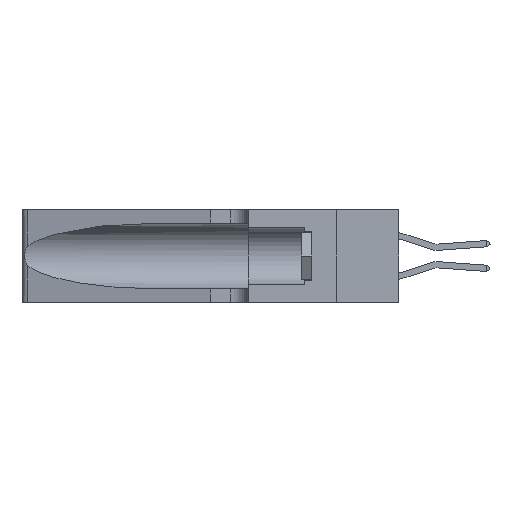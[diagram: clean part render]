
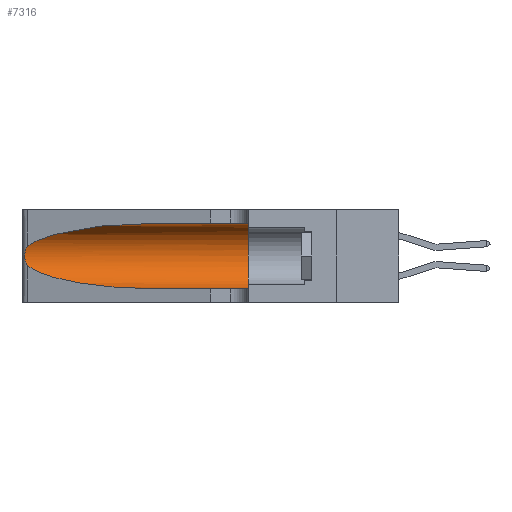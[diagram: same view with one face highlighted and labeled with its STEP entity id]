
A CAD part, left-side view. The second image highlights one B-rep face of the part: STEP entity #7316.
In plain terms, the highlighted cylindrical face has radius 3.308 mm (diameter 6.617 mm), a partial arc.
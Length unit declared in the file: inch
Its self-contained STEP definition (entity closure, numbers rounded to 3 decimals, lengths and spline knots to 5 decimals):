
#1073 = ORIENTED_EDGE ( 'NONE', *, *, #15432, .T. ) ;
#1999 = CARTESIAN_POINT ( 'NONE',  ( 0.25639, 1.23184, 0.21858 ) ) ;
#2359 = VERTEX_POINT ( 'NONE', #31182 ) ;
#3032 = EDGE_CURVE ( 'NONE', #23920, #23145, #36946, .T. ) ;
#3765 = EDGE_LOOP ( 'NONE', ( #6190, #25826, #1073, #31989, #12684, #25372 ) ) ;
#3889 = VERTEX_POINT ( 'NONE', #22416 ) ;
#5883 = LINE ( 'NONE', #26950, #29682 ) ;
#6063 = VERTEX_POINT ( 'NONE', #15982 ) ;
#6190 = ORIENTED_EDGE ( 'NONE', *, *, #37031, .T. ) ;
#7149 = CARTESIAN_POINT ( 'NONE',  ( 0.18966, 0.96281, 0.31525 ) ) ;
#7316 = ADVANCED_FACE ( 'NONE', ( #28765 ), #9544, .F. ) ;
#7388 = EDGE_CURVE ( 'NONE', #2359, #3889, #32401, .T. ) ;
#7562 = CARTESIAN_POINT ( 'NONE',  ( 0.1305, 0.35, 0.31525 ) ) ;
#7733 = DIRECTION ( 'NONE',  ( 0., -1., 0. ) ) ;
#7851 = CARTESIAN_POINT ( 'NONE',  ( 0.25555, 1.22993, 0.14849 ) ) ;
#8234 = CARTESIAN_POINT ( 'NONE',  ( 0.25789, 1.23486, 0.15765 ) ) ;
#9544 = CYLINDRICAL_SURFACE ( 'NONE', #13795, 0.13025 ) ;
#12684 = ORIENTED_EDGE ( 'NONE', *, *, #17105, .F. ) ;
#12778 = CARTESIAN_POINT ( 'NONE',  ( 0.1305, 0.72297, 0.05475 ) ) ;
#13628 = CARTESIAN_POINT ( 'NONE',  ( 0.25555, 1.22994, 0.2215 ) ) ;
#13795 = AXIS2_PLACEMENT_3D ( 'NONE', #34071, #28442, #22559 ) ;
#14013 = CARTESIAN_POINT ( 'NONE',  ( 0.25856, 1.23593, 0.16098 ) ) ;
#14461 = CIRCLE ( 'NONE', #29503, 0.13025 ) ;
#15432 = EDGE_CURVE ( 'NONE', #23145, #2359, #31832, .T. ) ;
#15732 = DIRECTION ( 'NONE',  ( 0., 0., 1. ) ) ;
#15753 = CARTESIAN_POINT ( 'NONE',  ( 0.2373, 1.15595, 0.28018 ) ) ;
#15982 = CARTESIAN_POINT ( 'NONE',  ( 0.1305, 0.72297, 0.31525 ) ) ;
#16129 = CARTESIAN_POINT ( 'NONE',  ( 0.18966, 0.96281, 0.05475 ) ) ;
#16344 = CARTESIAN_POINT ( 'NONE',  ( 0.1305, 1.61858, 0.05475 ) ) ;
#16713 = CARTESIAN_POINT ( 'NONE',  ( 0.26018, 1.23835, 0.19895 ) ) ;
#16841 = CARTESIAN_POINT ( 'NONE',  ( 0.26075, 1.23896, 0.178 ) ) ;
#16962 = CARTESIAN_POINT ( 'NONE',  ( 0.26075, 1.23896, 0.19203 ) ) ;
#17105 = EDGE_CURVE ( 'NONE', #30983, #3889, #14461, .T. ) ;
#19763 = CARTESIAN_POINT ( 'NONE',  ( 0.26017, 1.23833, 0.17102 ) ) ;
#19893 = CARTESIAN_POINT ( 'NONE',  ( 0.25639, 1.23186, 0.15144 ) ) ;
#21336 = DIRECTION ( 'NONE',  ( 0., 1., 0. ) ) ;
#21613 = CARTESIAN_POINT ( 'NONE',  ( 0.2373, 1.15595, 0.08982 ) ) ;
#22161 = EDGE_CURVE ( 'NONE', #6063, #30983, #5883, .T. ) ;
#22416 = CARTESIAN_POINT ( 'NONE',  ( 0.1305, 0.35, 0.05475 ) ) ;
#22559 = DIRECTION ( 'NONE',  ( 0., 0., -1. ) ) ;
#22684 = CARTESIAN_POINT ( 'NONE',  ( 0.25487, 1.22718, 0.14631 ) ) ;
#23145 = VERTEX_POINT ( 'NONE', #34272 ) ;
#23920 = VERTEX_POINT ( 'NONE', #29939 ) ;
#24531 = CARTESIAN_POINT ( 'NONE',  ( 0.25487, 1.22718, 0.22369 ) ) ;
#25372 = ORIENTED_EDGE ( 'NONE', *, *, #22161, .F. ) ;
#25826 = ORIENTED_EDGE ( 'NONE', *, *, #3032, .T. ) ;
#26182 =( BOUNDED_CURVE ( )  B_SPLINE_CURVE ( 3, ( #33111, #7149, #15753, #24531 ),
 .UNSPECIFIED., .F., .T. ) 
 B_SPLINE_CURVE_WITH_KNOTS ( ( 4, 4 ),
 ( 1.5708, 2.84003 ),
 .UNSPECIFIED. ) 
 CURVE ( )  GEOMETRIC_REPRESENTATION_ITEM ( )  RATIONAL_B_SPLINE_CURVE ( ( 1., 0.87, 0.87, 1. ) ) 
 REPRESENTATION_ITEM ( '' )  );
#26950 = CARTESIAN_POINT ( 'NONE',  ( 0.1305, 1.61858, 0.31525 ) ) ;
#28170 = CARTESIAN_POINT ( 'NONE',  ( 0.25487, 1.22718, 0.22369 ) ) ;
#28434 = CARTESIAN_POINT ( 'NONE',  ( 0.25854, 1.2359, 0.20912 ) ) ;
#28442 = DIRECTION ( 'NONE',  ( 0., -1., 0. ) ) ;
#28765 = FACE_OUTER_BOUND ( 'NONE', #3765, .T. ) ;
#29503 = AXIS2_PLACEMENT_3D ( 'NONE', #35745, #21336, #15732 ) ;
#29659 = VECTOR ( 'NONE', #7733, 39.37008 ) ;
#29682 = VECTOR ( 'NONE', #30056, 39.37008 ) ;
#29939 = CARTESIAN_POINT ( 'NONE',  ( 0.25487, 1.22718, 0.22369 ) ) ;
#30056 = DIRECTION ( 'NONE',  ( 0., -1., 0. ) ) ;
#30983 = VERTEX_POINT ( 'NONE', #7562 ) ;
#31182 = CARTESIAN_POINT ( 'NONE',  ( 0.1305, 0.72297, 0.05475 ) ) ;
#31512 = CARTESIAN_POINT ( 'NONE',  ( 0.25787, 1.23484, 0.2124 ) ) ;
#31832 =( BOUNDED_CURVE ( )  B_SPLINE_CURVE ( 3, ( #33601, #21613, #16129, #12778 ),
 .UNSPECIFIED., .F., .T. ) 
 B_SPLINE_CURVE_WITH_KNOTS ( ( 4, 4 ),
 ( 3.44316, 4.71239 ),
 .UNSPECIFIED. ) 
 CURVE ( )  GEOMETRIC_REPRESENTATION_ITEM ( )  RATIONAL_B_SPLINE_CURVE ( ( 1., 0.87, 0.87, 1. ) ) 
 REPRESENTATION_ITEM ( '' )  );
#31989 = ORIENTED_EDGE ( 'NONE', *, *, #7388, .T. ) ;
#32401 = LINE ( 'NONE', #16344, #29659 ) ;
#33111 = CARTESIAN_POINT ( 'NONE',  ( 0.1305, 0.72297, 0.31525 ) ) ;
#33601 = CARTESIAN_POINT ( 'NONE',  ( 0.25487, 1.22718, 0.14631 ) ) ;
#34071 = CARTESIAN_POINT ( 'NONE',  ( 0.1305, 1.61858, 0.185 ) ) ;
#34272 = CARTESIAN_POINT ( 'NONE',  ( 0.25487, 1.22718, 0.14631 ) ) ;
#35745 = CARTESIAN_POINT ( 'NONE',  ( 0.1305, 0.35, 0.185 ) ) ;
#36946 = B_SPLINE_CURVE_WITH_KNOTS ( 'NONE', 3,
 ( #28170, #13628, #1999, #31512, #28434, #16713, #16962, #16841, #19763, #14013, #8234, #19893, #7851, #22684 ),
 .UNSPECIFIED., .F., .F.,
 ( 4, 2, 2, 2, 2, 2, 4 ),
 ( 0., 0.00027, 0.00053, 0.00107, 0.0016, 0.00187, 0.00214 ),
 .UNSPECIFIED. ) ;
#37031 = EDGE_CURVE ( 'NONE', #6063, #23920, #26182, .T. ) ;
